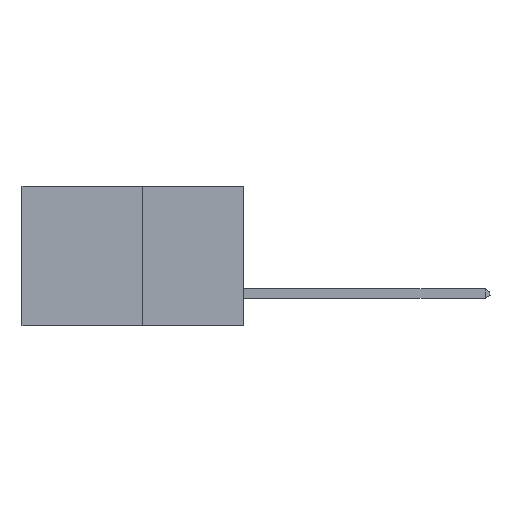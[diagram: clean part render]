
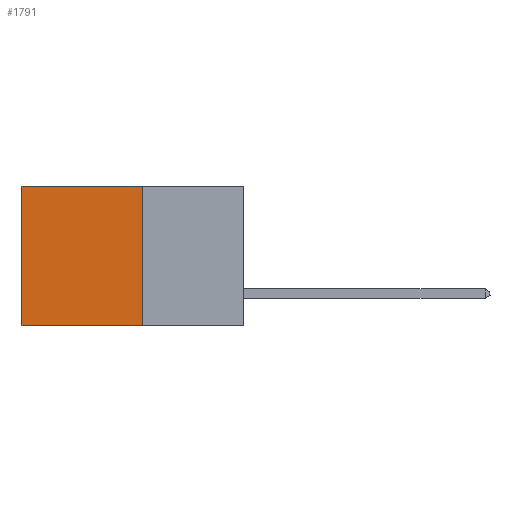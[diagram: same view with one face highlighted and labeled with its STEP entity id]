
A CAD part, left-side view. The second image highlights one B-rep face of the part: STEP entity #1791.
In plain terms, the highlighted planar face has unit normal (-1, 0, 0).
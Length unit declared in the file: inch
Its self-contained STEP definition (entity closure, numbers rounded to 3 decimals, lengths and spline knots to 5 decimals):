
#614 = DIRECTION ( 'NONE',  ( 0., 0., -1. ) ) ;
#920 = LINE ( 'NONE', #2700, #11431 ) ;
#977 = VECTOR ( 'NONE', #11926, 39.37008 ) ;
#1167 = DIRECTION ( 'NONE',  ( 1., 0., 0. ) ) ;
#1338 = CARTESIAN_POINT ( 'NONE',  ( 0.277, 0.59, -0.37 ) ) ;
#1590 = CARTESIAN_POINT ( 'NONE',  ( 0.277, 0.27, -0.37 ) ) ;
#1681 = DIRECTION ( 'NONE',  ( 0., 0., -1. ) ) ;
#1791 = ADVANCED_FACE ( 'NONE', ( #9453 ), #10724, .F. ) ;
#1920 = CARTESIAN_POINT ( 'NONE',  ( 0.277, 0.27, -0.37 ) ) ;
#2700 = CARTESIAN_POINT ( 'NONE',  ( 0.277, 0.59, -0.37 ) ) ;
#2722 = VERTEX_POINT ( 'NONE', #1338 ) ;
#2737 = CARTESIAN_POINT ( 'NONE',  ( 0.277, 0.27, -0.37 ) ) ;
#3671 = VERTEX_POINT ( 'NONE', #10220 ) ;
#3735 = LINE ( 'NONE', #11950, #9576 ) ;
#3975 = VERTEX_POINT ( 'NONE', #2737 ) ;
#4997 = AXIS2_PLACEMENT_3D ( 'NONE', #1920, #1167, #10739 ) ;
#5782 = ORIENTED_EDGE ( 'NONE', *, *, #12618, .F. ) ;
#6188 = EDGE_CURVE ( 'NONE', #3975, #2722, #11777, .T. ) ;
#6193 = EDGE_CURVE ( 'NONE', #3671, #11721, #3735, .T. ) ;
#6620 = EDGE_LOOP ( 'NONE', ( #7901, #10515, #5782, #12854 ) ) ;
#7901 = ORIENTED_EDGE ( 'NONE', *, *, #9015, .T. ) ;
#9015 = EDGE_CURVE ( 'NONE', #11721, #2722, #920, .T. ) ;
#9453 = FACE_OUTER_BOUND ( 'NONE', #6620, .T. ) ;
#9576 = VECTOR ( 'NONE', #11967, 39.37008 ) ;
#9585 = VECTOR ( 'NONE', #614, 39.37008 ) ;
#10220 = CARTESIAN_POINT ( 'NONE',  ( 0.277, 0.27, 0. ) ) ;
#10515 = ORIENTED_EDGE ( 'NONE', *, *, #6188, .F. ) ;
#10667 = CARTESIAN_POINT ( 'NONE',  ( 0.277, 0.59, 0. ) ) ;
#10724 = PLANE ( 'NONE',  #4997 ) ;
#10739 = DIRECTION ( 'NONE',  ( 0., 0., -1. ) ) ;
#11431 = VECTOR ( 'NONE', #1681, 39.37008 ) ;
#11721 = VERTEX_POINT ( 'NONE', #10667 ) ;
#11777 = LINE ( 'NONE', #12900, #977 ) ;
#11926 = DIRECTION ( 'NONE',  ( 0., 1., 0. ) ) ;
#11950 = CARTESIAN_POINT ( 'NONE',  ( 0.277, 0.27, 0. ) ) ;
#11967 = DIRECTION ( 'NONE',  ( 0., 1., 0. ) ) ;
#12066 = LINE ( 'NONE', #1590, #9585 ) ;
#12618 = EDGE_CURVE ( 'NONE', #3671, #3975, #12066, .T. ) ;
#12854 = ORIENTED_EDGE ( 'NONE', *, *, #6193, .T. ) ;
#12900 = CARTESIAN_POINT ( 'NONE',  ( 0.277, 0.27, -0.37 ) ) ;
